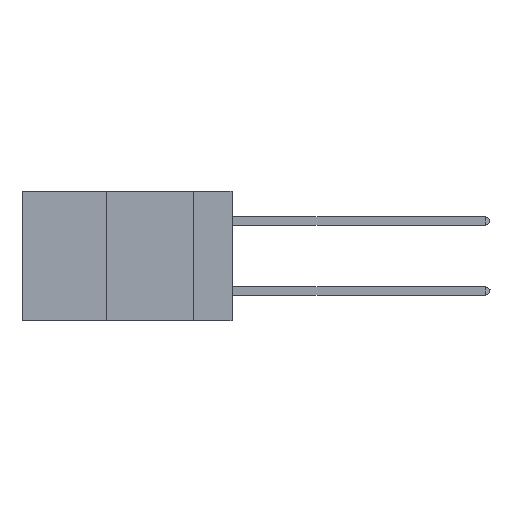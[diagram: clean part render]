
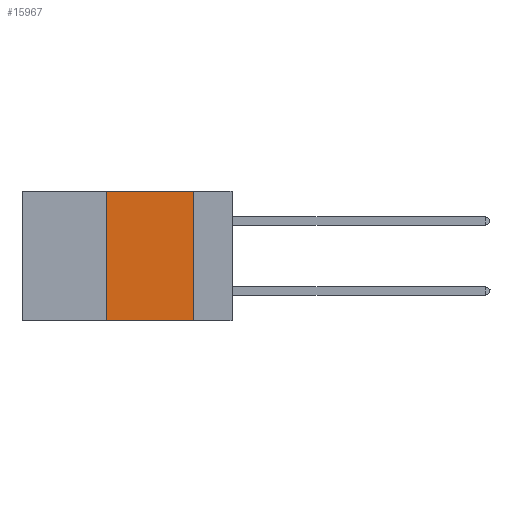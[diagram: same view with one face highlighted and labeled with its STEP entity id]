
A CAD part, left-side view. The second image highlights one B-rep face of the part: STEP entity #15967.
In plain terms, the highlighted planar face has unit normal (-1, 0, 0).
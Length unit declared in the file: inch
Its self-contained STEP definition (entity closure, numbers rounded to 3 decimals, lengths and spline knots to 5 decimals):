
#87 = ORIENTED_EDGE ( 'NONE', *, *, #17082, .T. ) ;
#1866 = PLANE ( 'NONE',  #16861 ) ;
#2219 = DIRECTION ( 'NONE',  ( 0., 0., 1. ) ) ;
#3586 = CARTESIAN_POINT ( 'NONE',  ( 0., 0.11, 0. ) ) ;
#4875 = CARTESIAN_POINT ( 'NONE',  ( 0., 0.6, -0.37 ) ) ;
#5058 = DIRECTION ( 'NONE',  ( 0., 0., -1. ) ) ;
#5276 = CARTESIAN_POINT ( 'NONE',  ( 0., 0.6, 0. ) ) ;
#5682 = CARTESIAN_POINT ( 'NONE',  ( 0., 0.36, 0. ) ) ;
#5690 = DIRECTION ( 'NONE',  ( 0., -1., 0. ) ) ;
#5801 = CARTESIAN_POINT ( 'NONE',  ( 0., 0.11, 0. ) ) ;
#9689 = ORIENTED_EDGE ( 'NONE', *, *, #17309, .F. ) ;
#10772 = CARTESIAN_POINT ( 'NONE',  ( 0., 0.11, -0.37 ) ) ;
#10942 = CARTESIAN_POINT ( 'NONE',  ( 0., 0.36, 0. ) ) ;
#12618 = EDGE_CURVE ( 'NONE', #22948, #33883, #39291, .T. ) ;
#13194 = LINE ( 'NONE', #3586, #17142 ) ;
#14166 = CARTESIAN_POINT ( 'NONE',  ( 0., 0.6, 0. ) ) ;
#15967 = ADVANCED_FACE ( 'NONE', ( #25675 ), #1866, .F. ) ;
#16073 = CARTESIAN_POINT ( 'NONE',  ( 0., 0.36, -0.37 ) ) ;
#16861 = AXIS2_PLACEMENT_3D ( 'NONE', #14166, #27290, #5058 ) ;
#17082 = EDGE_CURVE ( 'NONE', #18071, #20524, #38437, .T. ) ;
#17142 = VECTOR ( 'NONE', #31787, 39.37008 ) ;
#17309 = EDGE_CURVE ( 'NONE', #33883, #20524, #13194, .T. ) ;
#18071 = VERTEX_POINT ( 'NONE', #16073 ) ;
#20524 = VERTEX_POINT ( 'NONE', #10772 ) ;
#21921 = LINE ( 'NONE', #5682, #22930 ) ;
#22930 = VECTOR ( 'NONE', #2219, 39.37008 ) ;
#22948 = VERTEX_POINT ( 'NONE', #10942 ) ;
#25423 = EDGE_LOOP ( 'NONE', ( #9689, #34039, #28763, #87 ) ) ;
#25675 = FACE_OUTER_BOUND ( 'NONE', #25423, .T. ) ;
#27290 = DIRECTION ( 'NONE',  ( 1., 0., 0. ) ) ;
#27359 = DIRECTION ( 'NONE',  ( 0., -1., 0. ) ) ;
#28763 = ORIENTED_EDGE ( 'NONE', *, *, #30417, .F. ) ;
#30033 = VECTOR ( 'NONE', #5690, 39.37008 ) ;
#30417 = EDGE_CURVE ( 'NONE', #18071, #22948, #21921, .T. ) ;
#31787 = DIRECTION ( 'NONE',  ( 0., 0., -1. ) ) ;
#33883 = VERTEX_POINT ( 'NONE', #5801 ) ;
#34039 = ORIENTED_EDGE ( 'NONE', *, *, #12618, .F. ) ;
#38275 = VECTOR ( 'NONE', #27359, 39.37008 ) ;
#38437 = LINE ( 'NONE', #4875, #30033 ) ;
#39291 = LINE ( 'NONE', #5276, #38275 ) ;
